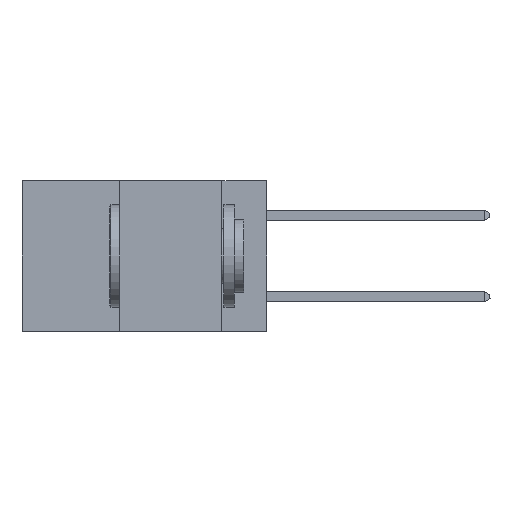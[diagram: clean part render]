
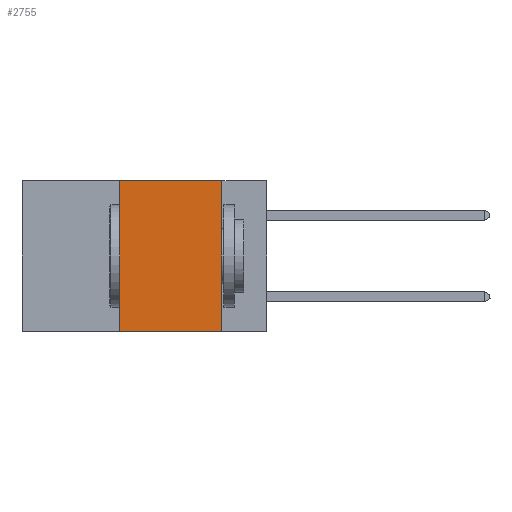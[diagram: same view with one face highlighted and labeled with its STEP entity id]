
A CAD part, left-side view. The second image highlights one B-rep face of the part: STEP entity #2755.
In plain terms, the highlighted planar face has unit normal (-1, 0, 0).
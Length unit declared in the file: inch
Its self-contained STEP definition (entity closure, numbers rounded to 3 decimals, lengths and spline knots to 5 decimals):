
#460 = VERTEX_POINT ( 'NONE', #5551 ) ;
#598 = CARTESIAN_POINT ( 'NONE',  ( 0., 0.6, -0.37 ) ) ;
#817 = VERTEX_POINT ( 'NONE', #3155 ) ;
#1461 = VECTOR ( 'NONE', #15346, 39.37008 ) ;
#1494 = FACE_OUTER_BOUND ( 'NONE', #8695, .T. ) ;
#1496 = EDGE_CURVE ( 'NONE', #460, #18012, #10575, .T. ) ;
#2297 = ORIENTED_EDGE ( 'NONE', *, *, #17114, .T. ) ;
#2755 = ADVANCED_FACE ( 'NONE', ( #1494 ), #4721, .F. ) ;
#2792 = ORIENTED_EDGE ( 'NONE', *, *, #15233, .F. ) ;
#3155 = CARTESIAN_POINT ( 'NONE',  ( 0., 0.36, -0.37 ) ) ;
#3442 = VECTOR ( 'NONE', #12660, 39.37008 ) ;
#3444 = DIRECTION ( 'NONE',  ( 0., 0., -1. ) ) ;
#3974 = CARTESIAN_POINT ( 'NONE',  ( 0., 0.36, 0. ) ) ;
#4083 = VECTOR ( 'NONE', #16041, 39.37008 ) ;
#4347 = LINE ( 'NONE', #16810, #1461 ) ;
#4721 = PLANE ( 'NONE',  #13059 ) ;
#4784 = DIRECTION ( 'NONE',  ( 1., 0., 0. ) ) ;
#5551 = CARTESIAN_POINT ( 'NONE',  ( 0., 0.36, 0. ) ) ;
#5623 = LINE ( 'NONE', #598, #4083 ) ;
#5673 = CARTESIAN_POINT ( 'NONE',  ( 0., 0.11, -0.37 ) ) ;
#7681 = CARTESIAN_POINT ( 'NONE',  ( 0., 0.6, 0. ) ) ;
#8260 = CARTESIAN_POINT ( 'NONE',  ( 0., 0.11, 0. ) ) ;
#8695 = EDGE_LOOP ( 'NONE', ( #2792, #12713, #11440, #2297 ) ) ;
#10282 = EDGE_CURVE ( 'NONE', #817, #460, #17445, .T. ) ;
#10575 = LINE ( 'NONE', #17998, #13777 ) ;
#11440 = ORIENTED_EDGE ( 'NONE', *, *, #10282, .F. ) ;
#11516 = DIRECTION ( 'NONE',  ( 0., -1., 0. ) ) ;
#11781 = VERTEX_POINT ( 'NONE', #5673 ) ;
#12660 = DIRECTION ( 'NONE',  ( 0., 0., 1. ) ) ;
#12713 = ORIENTED_EDGE ( 'NONE', *, *, #1496, .F. ) ;
#13059 = AXIS2_PLACEMENT_3D ( 'NONE', #7681, #4784, #3444 ) ;
#13777 = VECTOR ( 'NONE', #11516, 39.37008 ) ;
#15233 = EDGE_CURVE ( 'NONE', #18012, #11781, #4347, .T. ) ;
#15346 = DIRECTION ( 'NONE',  ( 0., 0., -1. ) ) ;
#16041 = DIRECTION ( 'NONE',  ( 0., -1., 0. ) ) ;
#16810 = CARTESIAN_POINT ( 'NONE',  ( 0., 0.11, 0. ) ) ;
#17114 = EDGE_CURVE ( 'NONE', #817, #11781, #5623, .T. ) ;
#17445 = LINE ( 'NONE', #3974, #3442 ) ;
#17998 = CARTESIAN_POINT ( 'NONE',  ( 0., 0.6, 0. ) ) ;
#18012 = VERTEX_POINT ( 'NONE', #8260 ) ;
